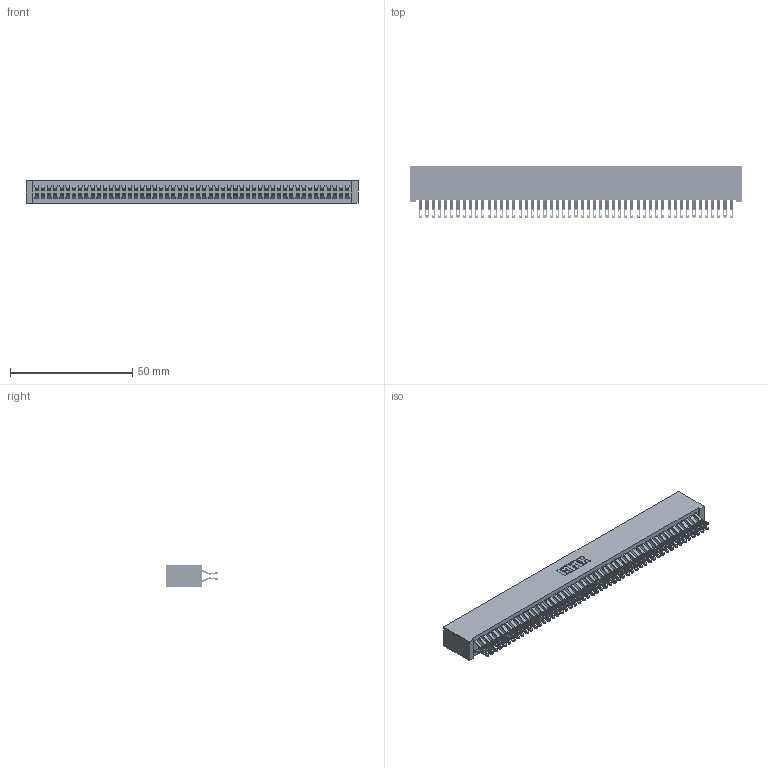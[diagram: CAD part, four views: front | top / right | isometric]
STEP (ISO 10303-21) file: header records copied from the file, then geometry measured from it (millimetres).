
FILE_DESCRIPTION (( 'STEP AP203' ), '1' );
FILE_NAME ('392-102-555-201.STEP', '2018-08-18T19:05:01', ( '' ), ( '' ), 'SwSTEP 2.0', 'SolidWorks 2016', '' );
FILE_SCHEMA (( 'CONFIG_CONTROL_DESIGN' ));
Length unit declared in the file: inch
Products named in the file (3): 342 Part_Lugless; 345-292-001_555 Tail; 392-102-555-201
Assembly tree (103 placements, depth 2):
  392-102-555-201
    342 Part_Lugless
    345-292-001_555 Tail  x102
Bounding box: 135.79 x 21.47 x 9.4 mm (x, y, z)
Volume: 12966.1 mm3; surface area: 22760.5 mm2
Topology: 103 solids, 103 shells, 6018 faces, 18941 edges, 12626 vertices
Faces by surface type: plane 3530, cylinder 2488
Entity records: 31563 total; most frequent: CARTESIAN_POINT 5252, ORIENTED_EDGE 5158, DIRECTION 4435, EDGE_CURVE 2579, VECTOR 2439, LINE 2439, VERTEX_POINT 1718, AXIS2_PLACEMENT_3D 998
